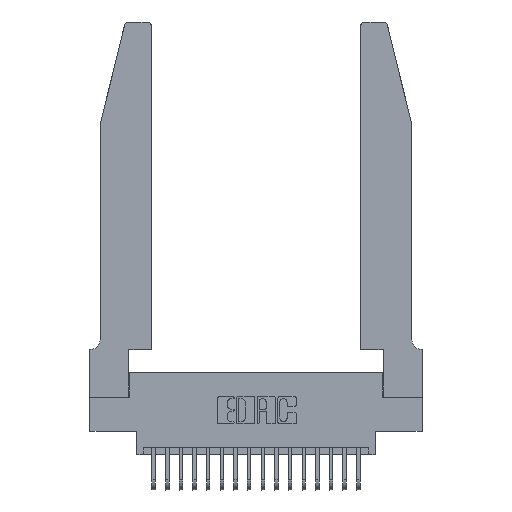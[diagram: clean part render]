
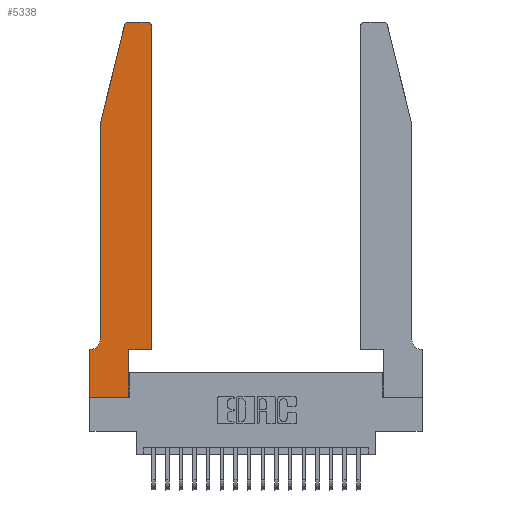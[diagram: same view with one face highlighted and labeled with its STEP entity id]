
A CAD part, top view. The second image highlights one B-rep face of the part: STEP entity #5338.
In plain terms, the highlighted planar face has unit normal (0, 0, 1).
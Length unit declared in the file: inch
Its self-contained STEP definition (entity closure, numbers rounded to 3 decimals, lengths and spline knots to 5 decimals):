
#316 = CIRCLE ( 'NONE', #13530, 0.03 ) ;
#720 = CARTESIAN_POINT ( 'NONE',  ( 0.2865, 0.35, 0.37 ) ) ;
#824 = CARTESIAN_POINT ( 'NONE',  ( 0.284, 2.75, 0.37 ) ) ;
#895 = CARTESIAN_POINT ( 'NONE',  ( 0.0055, 0.35, 0.37 ) ) ;
#953 = DIRECTION ( 'NONE',  ( 0., -1., 0. ) ) ;
#972 = DIRECTION ( 'NONE',  ( 0., 0., 1. ) ) ;
#1013 = EDGE_CURVE ( 'NONE', #20135, #11495, #20151, .T. ) ;
#1411 = DIRECTION ( 'NONE',  ( 1., 0., 0. ) ) ;
#1879 = DIRECTION ( 'NONE',  ( -1., 0., 0. ) ) ;
#2238 = AXIS2_PLACEMENT_3D ( 'NONE', #16235, #7632, #5720 ) ;
#2545 = VECTOR ( 'NONE', #16409, 39.37008 ) ;
#3042 = LINE ( 'NONE', #13975, #19990 ) ;
#3047 = DIRECTION ( 'NONE',  ( 0., -1., 0. ) ) ;
#3527 = LINE ( 'NONE', #5198, #21576 ) ;
#3852 = CARTESIAN_POINT ( 'NONE',  ( 0.0755, 2., 0.37 ) ) ;
#4143 = VECTOR ( 'NONE', #953, 39.37008 ) ;
#4308 = LINE ( 'NONE', #13171, #13857 ) ;
#4326 = EDGE_CURVE ( 'NONE', #6782, #16024, #12093, .T. ) ;
#4549 = EDGE_CURVE ( 'NONE', #14445, #10671, #316, .T. ) ;
#4777 = AXIS2_PLACEMENT_3D ( 'NONE', #18615, #972, #13409 ) ;
#5025 = EDGE_LOOP ( 'NONE', ( #12869, #6572, #10602, #11174, #5141, #14122, #18471, #17600, #6584, #8878, #7172, #13468 ) ) ;
#5141 = ORIENTED_EDGE ( 'NONE', *, *, #22297, .T. ) ;
#5198 = CARTESIAN_POINT ( 'NONE',  ( 0.2605, 2.75, 0.37 ) ) ;
#5338 = ADVANCED_FACE ( 'NONE', ( #7126 ), #7057, .T. ) ;
#5421 = VECTOR ( 'NONE', #17774, 39.37008 ) ;
#5720 = DIRECTION ( 'NONE',  ( 1., 0., 0. ) ) ;
#6572 = ORIENTED_EDGE ( 'NONE', *, *, #4549, .T. ) ;
#6584 = ORIENTED_EDGE ( 'NONE', *, *, #20805, .T. ) ;
#6782 = VERTEX_POINT ( 'NONE', #15347 ) ;
#7057 = PLANE ( 'NONE',  #4777 ) ;
#7126 = FACE_OUTER_BOUND ( 'NONE', #5025, .T. ) ;
#7172 = ORIENTED_EDGE ( 'NONE', *, *, #13932, .T. ) ;
#7277 = DIRECTION ( 'NONE',  ( 1., 0., 0. ) ) ;
#7617 = LINE ( 'NONE', #21237, #5421 ) ;
#7632 = DIRECTION ( 'NONE',  ( 0., 0., 1. ) ) ;
#7679 = VERTEX_POINT ( 'NONE', #12786 ) ;
#7734 = CARTESIAN_POINT ( 'NONE',  ( 0.0755, 2., 0.37 ) ) ;
#7891 = DIRECTION ( 'NONE',  ( 1., 0., 0. ) ) ;
#7962 = LINE ( 'NONE', #11823, #10946 ) ;
#7994 = LINE ( 'NONE', #7734, #17023 ) ;
#8878 = ORIENTED_EDGE ( 'NONE', *, *, #22412, .T. ) ;
#9011 = DIRECTION ( 'NONE',  ( 0., 0., -1. ) ) ;
#9238 = CARTESIAN_POINT ( 'NONE',  ( 0.0055, 0.42, 0.37 ) ) ;
#9770 = EDGE_CURVE ( 'NONE', #13182, #20135, #19454, .T. ) ;
#10202 = DIRECTION ( 'NONE',  ( 0., 0., 1. ) ) ;
#10602 = ORIENTED_EDGE ( 'NONE', *, *, #13059, .T. ) ;
#10671 = VERTEX_POINT ( 'NONE', #14178 ) ;
#10946 = VECTOR ( 'NONE', #3047, 39.37008 ) ;
#11174 = ORIENTED_EDGE ( 'NONE', *, *, #14180, .T. ) ;
#11269 = VERTEX_POINT ( 'NONE', #895 ) ;
#11495 = VERTEX_POINT ( 'NONE', #15756 ) ;
#11823 = CARTESIAN_POINT ( 'NONE',  ( 0.0755, 2., 0.37 ) ) ;
#11955 = CARTESIAN_POINT ( 'NONE',  ( 0.284, 2.72, 0.37 ) ) ;
#12093 = CIRCLE ( 'NONE', #2238, 0.03 ) ;
#12439 = DIRECTION ( 'NONE',  ( 0., 1., 0. ) ) ;
#12460 = CARTESIAN_POINT ( 'NONE',  ( 0., 0., 0.37 ) ) ;
#12468 = VECTOR ( 'NONE', #7277, 39.37008 ) ;
#12786 = CARTESIAN_POINT ( 'NONE',  ( 0.0755, 0.42, 0.37 ) ) ;
#12852 = DIRECTION ( 'NONE',  ( -0.239, -0.971, 0. ) ) ;
#12869 = ORIENTED_EDGE ( 'NONE', *, *, #20751, .T. ) ;
#13059 = EDGE_CURVE ( 'NONE', #10671, #22203, #7994, .T. ) ;
#13171 = CARTESIAN_POINT ( 'NONE',  ( 0.4505, 0.35, 0.37 ) ) ;
#13182 = VERTEX_POINT ( 'NONE', #18747 ) ;
#13409 = DIRECTION ( 'NONE',  ( 1., 0., 0. ) ) ;
#13468 = ORIENTED_EDGE ( 'NONE', *, *, #4326, .T. ) ;
#13530 = AXIS2_PLACEMENT_3D ( 'NONE', #11955, #10202, #1411 ) ;
#13857 = VECTOR ( 'NONE', #7891, 39.37008 ) ;
#13932 = EDGE_CURVE ( 'NONE', #14173, #6782, #3042, .T. ) ;
#13975 = CARTESIAN_POINT ( 'NONE',  ( 0.4505, 0.35, 0.37 ) ) ;
#14122 = ORIENTED_EDGE ( 'NONE', *, *, #18798, .T. ) ;
#14173 = VERTEX_POINT ( 'NONE', #15402 ) ;
#14178 = CARTESIAN_POINT ( 'NONE',  ( 0.25487, 2.72718, 0.37 ) ) ;
#14180 = EDGE_CURVE ( 'NONE', #22203, #7679, #7962, .T. ) ;
#14196 = CARTESIAN_POINT ( 'NONE',  ( 0., 0., 0.37 ) ) ;
#14445 = VERTEX_POINT ( 'NONE', #824 ) ;
#14801 = CARTESIAN_POINT ( 'NONE',  ( 0.0755, 0.35, 0.37 ) ) ;
#15347 = CARTESIAN_POINT ( 'NONE',  ( 0.4505, 2.72, 0.37 ) ) ;
#15402 = CARTESIAN_POINT ( 'NONE',  ( 0.4505, 0.35, 0.37 ) ) ;
#15756 = CARTESIAN_POINT ( 'NONE',  ( 0.2865, 0., 0.37 ) ) ;
#16024 = VERTEX_POINT ( 'NONE', #21003 ) ;
#16235 = CARTESIAN_POINT ( 'NONE',  ( 0.4205, 2.72, 0.37 ) ) ;
#16409 = DIRECTION ( 'NONE',  ( -1., 0., 0. ) ) ;
#17023 = VECTOR ( 'NONE', #12852, 39.37008 ) ;
#17600 = ORIENTED_EDGE ( 'NONE', *, *, #1013, .T. ) ;
#17774 = DIRECTION ( 'NONE',  ( 0., 1., 0. ) ) ;
#17846 = LINE ( 'NONE', #14801, #2545 ) ;
#18029 = AXIS2_PLACEMENT_3D ( 'NONE', #9238, #9011, #21280 ) ;
#18212 = VERTEX_POINT ( 'NONE', #720 ) ;
#18471 = ORIENTED_EDGE ( 'NONE', *, *, #9770, .T. ) ;
#18615 = CARTESIAN_POINT ( 'NONE',  ( 0., 0.35, 0.37 ) ) ;
#18747 = CARTESIAN_POINT ( 'NONE',  ( 0., 0.35, 0.37 ) ) ;
#18798 = EDGE_CURVE ( 'NONE', #11269, #13182, #17846, .T. ) ;
#19454 = LINE ( 'NONE', #21216, #4143 ) ;
#19990 = VECTOR ( 'NONE', #12439, 39.37008 ) ;
#20135 = VERTEX_POINT ( 'NONE', #12460 ) ;
#20151 = LINE ( 'NONE', #14196, #12468 ) ;
#20721 = CIRCLE ( 'NONE', #18029, 0.07 ) ;
#20751 = EDGE_CURVE ( 'NONE', #16024, #14445, #3527, .T. ) ;
#20805 = EDGE_CURVE ( 'NONE', #11495, #18212, #7617, .T. ) ;
#21003 = CARTESIAN_POINT ( 'NONE',  ( 0.4205, 2.75, 0.37 ) ) ;
#21216 = CARTESIAN_POINT ( 'NONE',  ( 0., 0., 0.37 ) ) ;
#21237 = CARTESIAN_POINT ( 'NONE',  ( 0.2865, 0.35, 0.37 ) ) ;
#21280 = DIRECTION ( 'NONE',  ( -1., 0., 0. ) ) ;
#21576 = VECTOR ( 'NONE', #1879, 39.37008 ) ;
#22203 = VERTEX_POINT ( 'NONE', #3852 ) ;
#22297 = EDGE_CURVE ( 'NONE', #7679, #11269, #20721, .T. ) ;
#22412 = EDGE_CURVE ( 'NONE', #18212, #14173, #4308, .T. ) ;
